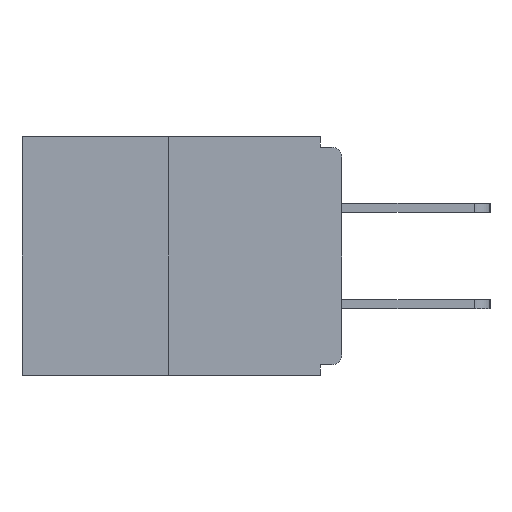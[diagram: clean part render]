
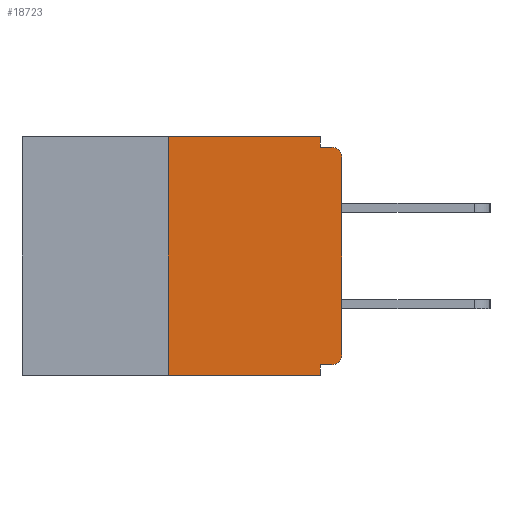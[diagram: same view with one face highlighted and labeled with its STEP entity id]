
A CAD part, left-side view. The second image highlights one B-rep face of the part: STEP entity #18723.
In plain terms, the highlighted planar face has unit normal (-1, 0, 0).
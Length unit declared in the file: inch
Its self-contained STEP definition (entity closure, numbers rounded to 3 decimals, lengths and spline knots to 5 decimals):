
#266 = VERTEX_POINT ( 'NONE', #20861 ) ;
#406 = CARTESIAN_POINT ( 'NONE',  ( 0., 0., -0.313 ) ) ;
#526 = DIRECTION ( 'NONE',  ( 0., 0., -1. ) ) ;
#1130 = ORIENTED_EDGE ( 'NONE', *, *, #21780, .F. ) ;
#1206 = VERTEX_POINT ( 'NONE', #3428 ) ;
#1738 = VECTOR ( 'NONE', #5550, 39.37008 ) ;
#1810 = VERTEX_POINT ( 'NONE', #406 ) ;
#2123 = EDGE_CURVE ( 'NONE', #16109, #9086, #7210, .T. ) ;
#2362 = CARTESIAN_POINT ( 'NONE',  ( 0., 0.031, -0.343 ) ) ;
#2441 = EDGE_CURVE ( 'NONE', #1206, #9086, #6355, .T. ) ;
#2851 = LINE ( 'NONE', #20226, #11152 ) ;
#3088 = CARTESIAN_POINT ( 'NONE',  ( 0., 0.25, 0. ) ) ;
#3261 = DIRECTION ( 'NONE',  ( 0., 0., -1. ) ) ;
#3317 = VECTOR ( 'NONE', #8702, 39.37008 ) ;
#3340 = DIRECTION ( 'NONE',  ( 0., 0., -1. ) ) ;
#3399 = AXIS2_PLACEMENT_3D ( 'NONE', #5046, #20830, #3340 ) ;
#3416 = CARTESIAN_POINT ( 'NONE',  ( 0., 0.015, -0.03 ) ) ;
#3422 = CARTESIAN_POINT ( 'NONE',  ( 0., 0.25, -0.343 ) ) ;
#3428 = CARTESIAN_POINT ( 'NONE',  ( 0., 0., -0.03 ) ) ;
#3485 = FACE_OUTER_BOUND ( 'NONE', #11081, .T. ) ;
#3865 = VERTEX_POINT ( 'NONE', #3422 ) ;
#4067 = LINE ( 'NONE', #2362, #18408 ) ;
#4427 = EDGE_CURVE ( 'NONE', #1810, #1206, #8890, .T. ) ;
#4443 = DIRECTION ( 'NONE',  ( 0., -1., 0. ) ) ;
#4904 = ORIENTED_EDGE ( 'NONE', *, *, #2441, .T. ) ;
#5046 = CARTESIAN_POINT ( 'NONE',  ( 0., 0.015, -0.313 ) ) ;
#5423 = DIRECTION ( 'NONE',  ( 1., 0., 0. ) ) ;
#5550 = DIRECTION ( 'NONE',  ( 0., 1., 0. ) ) ;
#5798 = ORIENTED_EDGE ( 'NONE', *, *, #22720, .F. ) ;
#6294 = ORIENTED_EDGE ( 'NONE', *, *, #16688, .F. ) ;
#6324 = VECTOR ( 'NONE', #11889, 39.37008 ) ;
#6355 = CIRCLE ( 'NONE', #7094, 0.015 ) ;
#6603 = DIRECTION ( 'NONE',  ( 0., 0., -1. ) ) ;
#6925 = VECTOR ( 'NONE', #3261, 39.37008 ) ;
#6959 = VERTEX_POINT ( 'NONE', #8369 ) ;
#6977 = DIRECTION ( 'NONE',  ( 0., 0., 1. ) ) ;
#7039 = CARTESIAN_POINT ( 'NONE',  ( 0., 0., 0. ) ) ;
#7094 = AXIS2_PLACEMENT_3D ( 'NONE', #3416, #15487, #6603 ) ;
#7210 = LINE ( 'NONE', #14374, #10866 ) ;
#7255 = CARTESIAN_POINT ( 'NONE',  ( 0., 0., -0.328 ) ) ;
#7357 = CARTESIAN_POINT ( 'NONE',  ( 0., 0.46, 0. ) ) ;
#7508 = VERTEX_POINT ( 'NONE', #8578 ) ;
#8290 = CARTESIAN_POINT ( 'NONE',  ( 0., 0.25, 0. ) ) ;
#8369 = CARTESIAN_POINT ( 'NONE',  ( 0., 0.031, 0. ) ) ;
#8578 = CARTESIAN_POINT ( 'NONE',  ( 0., 0.015, -0.328 ) ) ;
#8702 = DIRECTION ( 'NONE',  ( 0., -1., 0. ) ) ;
#8890 = LINE ( 'NONE', #7039, #6324 ) ;
#8928 = LINE ( 'NONE', #15956, #3317 ) ;
#9086 = VERTEX_POINT ( 'NONE', #9290 ) ;
#9290 = CARTESIAN_POINT ( 'NONE',  ( 0., 0.015, -0.015 ) ) ;
#9358 = EDGE_CURVE ( 'NONE', #3865, #22650, #8928, .T. ) ;
#10261 = VERTEX_POINT ( 'NONE', #8290 ) ;
#10311 = LINE ( 'NONE', #3088, #19486 ) ;
#10610 = ORIENTED_EDGE ( 'NONE', *, *, #2123, .F. ) ;
#10678 = DIRECTION ( 'NONE',  ( 0., -1., 0. ) ) ;
#10866 = VECTOR ( 'NONE', #10678, 39.37008 ) ;
#11081 = EDGE_LOOP ( 'NONE', ( #12078, #1130, #14695, #5798, #6294, #11223, #17427, #4904, #10610, #18450 ) ) ;
#11152 = VECTOR ( 'NONE', #4443, 39.37008 ) ;
#11223 = ORIENTED_EDGE ( 'NONE', *, *, #11537, .T. ) ;
#11537 = EDGE_CURVE ( 'NONE', #7508, #1810, #20672, .T. ) ;
#11889 = DIRECTION ( 'NONE',  ( 0., 0., 1. ) ) ;
#12078 = ORIENTED_EDGE ( 'NONE', *, *, #13393, .F. ) ;
#12440 = DIRECTION ( 'NONE',  ( 0., 0., -1. ) ) ;
#13393 = EDGE_CURVE ( 'NONE', #10261, #6959, #2851, .T. ) ;
#14374 = CARTESIAN_POINT ( 'NONE',  ( 0., 0., -0.015 ) ) ;
#14695 = ORIENTED_EDGE ( 'NONE', *, *, #9358, .T. ) ;
#15487 = DIRECTION ( 'NONE',  ( -1., 0., 0. ) ) ;
#15935 = CARTESIAN_POINT ( 'NONE',  ( 0., 0.031, -0.343 ) ) ;
#15956 = CARTESIAN_POINT ( 'NONE',  ( 0., 0.46, -0.343 ) ) ;
#16109 = VERTEX_POINT ( 'NONE', #20661 ) ;
#16508 = LINE ( 'NONE', #19478, #6925 ) ;
#16688 = EDGE_CURVE ( 'NONE', #7508, #266, #19143, .T. ) ;
#17427 = ORIENTED_EDGE ( 'NONE', *, *, #4427, .T. ) ;
#17629 = PLANE ( 'NONE',  #19019 ) ;
#18408 = VECTOR ( 'NONE', #526, 39.37008 ) ;
#18450 = ORIENTED_EDGE ( 'NONE', *, *, #20902, .F. ) ;
#18723 = ADVANCED_FACE ( 'NONE', ( #3485 ), #17629, .F. ) ;
#19019 = AXIS2_PLACEMENT_3D ( 'NONE', #7357, #5423, #12440 ) ;
#19143 = LINE ( 'NONE', #7255, #1738 ) ;
#19478 = CARTESIAN_POINT ( 'NONE',  ( 0., 0.031, 0. ) ) ;
#19486 = VECTOR ( 'NONE', #6977, 39.37008 ) ;
#20226 = CARTESIAN_POINT ( 'NONE',  ( 0., 0.46, 0. ) ) ;
#20661 = CARTESIAN_POINT ( 'NONE',  ( 0., 0.031, -0.015 ) ) ;
#20672 = CIRCLE ( 'NONE', #3399, 0.015 ) ;
#20830 = DIRECTION ( 'NONE',  ( -1., 0., 0. ) ) ;
#20861 = CARTESIAN_POINT ( 'NONE',  ( 0., 0.031, -0.328 ) ) ;
#20902 = EDGE_CURVE ( 'NONE', #6959, #16109, #16508, .T. ) ;
#21780 = EDGE_CURVE ( 'NONE', #3865, #10261, #10311, .T. ) ;
#22650 = VERTEX_POINT ( 'NONE', #15935 ) ;
#22720 = EDGE_CURVE ( 'NONE', #266, #22650, #4067, .T. ) ;
